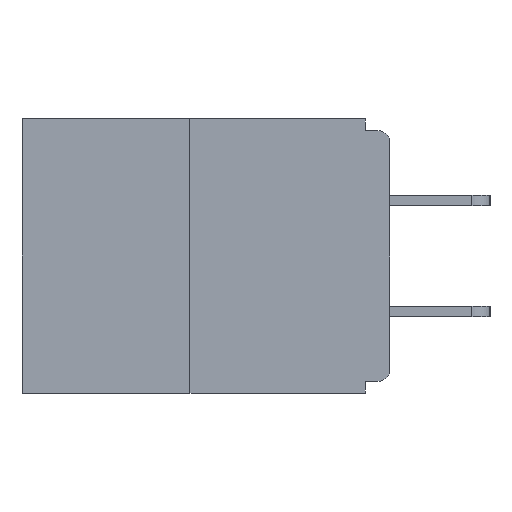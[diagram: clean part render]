
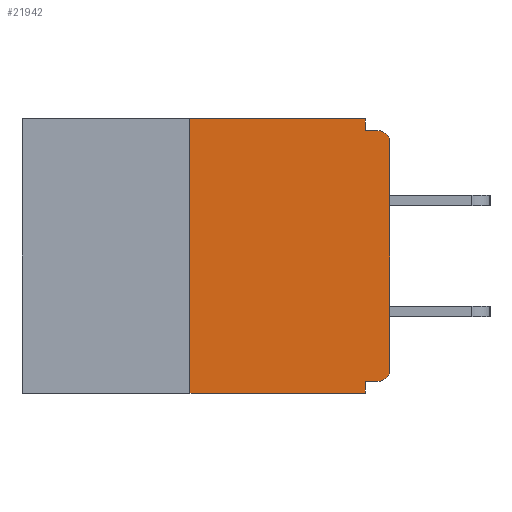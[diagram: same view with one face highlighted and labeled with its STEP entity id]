
A CAD part, left-side view. The second image highlights one B-rep face of the part: STEP entity #21942.
In plain terms, the highlighted planar face has unit normal (-1, 0, 0).
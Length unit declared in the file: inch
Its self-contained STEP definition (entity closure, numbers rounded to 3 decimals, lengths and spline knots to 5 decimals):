
#361 = VERTEX_POINT ( 'NONE', #21923 ) ;
#434 = VERTEX_POINT ( 'NONE', #30134 ) ;
#454 = ORIENTED_EDGE ( 'NONE', *, *, #24535, .T. ) ;
#1662 = ORIENTED_EDGE ( 'NONE', *, *, #8496, .T. ) ;
#2709 = EDGE_CURVE ( 'NONE', #361, #27647, #26786, .T. ) ;
#2742 = DIRECTION ( 'NONE',  ( 0., -1., 0. ) ) ;
#3403 = CARTESIAN_POINT ( 'NONE',  ( 0., 0.25, 0. ) ) ;
#4542 = VECTOR ( 'NONE', #15902, 39.37008 ) ;
#4855 = DIRECTION ( 'NONE',  ( 0., -1., 0. ) ) ;
#4894 = EDGE_CURVE ( 'NONE', #434, #29636, #6493, .T. ) ;
#4909 = DIRECTION ( 'NONE',  ( 0., 0., 1. ) ) ;
#4997 = VECTOR ( 'NONE', #4909, 39.37008 ) ;
#5574 = DIRECTION ( 'NONE',  ( 0., 0., -1. ) ) ;
#5601 = AXIS2_PLACEMENT_3D ( 'NONE', #25874, #28331, #13828 ) ;
#5640 = LINE ( 'NONE', #29507, #22577 ) ;
#5735 = ORIENTED_EDGE ( 'NONE', *, *, #2709, .F. ) ;
#6018 = VERTEX_POINT ( 'NONE', #18934 ) ;
#6100 = CARTESIAN_POINT ( 'NONE',  ( 0., 0.031, -0.343 ) ) ;
#6493 = LINE ( 'NONE', #15748, #4542 ) ;
#6708 = VECTOR ( 'NONE', #10724, 39.37008 ) ;
#7488 = VECTOR ( 'NONE', #20010, 39.37008 ) ;
#7684 = CARTESIAN_POINT ( 'NONE',  ( 0., 0.25, 0. ) ) ;
#8496 = EDGE_CURVE ( 'NONE', #24324, #27647, #19234, .T. ) ;
#10557 = EDGE_CURVE ( 'NONE', #6018, #22623, #15461, .T. ) ;
#10595 = CARTESIAN_POINT ( 'NONE',  ( 0., 0., 0. ) ) ;
#10724 = DIRECTION ( 'NONE',  ( 0., 0., -1. ) ) ;
#10898 = ORIENTED_EDGE ( 'NONE', *, *, #10557, .T. ) ;
#11642 = FACE_OUTER_BOUND ( 'NONE', #13571, .T. ) ;
#12263 = DIRECTION ( 'NONE',  ( 1., 0., 0. ) ) ;
#12884 = DIRECTION ( 'NONE',  ( 0., -1., 0. ) ) ;
#13135 = CARTESIAN_POINT ( 'NONE',  ( 0., 0.031, -0.015 ) ) ;
#13571 = EDGE_LOOP ( 'NONE', ( #16494, #15520, #1662, #5735, #25072, #22293, #454, #10898, #22321, #21813 ) ) ;
#13828 = DIRECTION ( 'NONE',  ( 0., 0., -1. ) ) ;
#13942 = CARTESIAN_POINT ( 'NONE',  ( 0., 0.46, 0. ) ) ;
#14294 = CARTESIAN_POINT ( 'NONE',  ( 0., 0.25, -0.343 ) ) ;
#14416 = PLANE ( 'NONE',  #18650 ) ;
#15041 = DIRECTION ( 'NONE',  ( 0., 1., 0. ) ) ;
#15461 = CIRCLE ( 'NONE', #5601, 0.015 ) ;
#15520 = ORIENTED_EDGE ( 'NONE', *, *, #24374, .F. ) ;
#15748 = CARTESIAN_POINT ( 'NONE',  ( 0., 0.031, 0. ) ) ;
#15755 = EDGE_CURVE ( 'NONE', #24033, #434, #21668, .T. ) ;
#15902 = DIRECTION ( 'NONE',  ( 0., 0., -1. ) ) ;
#16403 = EDGE_CURVE ( 'NONE', #29307, #30329, #26588, .T. ) ;
#16494 = ORIENTED_EDGE ( 'NONE', *, *, #15755, .F. ) ;
#16725 = DIRECTION ( 'NONE',  ( 0., 0., -1. ) ) ;
#17260 = VECTOR ( 'NONE', #4855, 39.37008 ) ;
#17502 = CARTESIAN_POINT ( 'NONE',  ( 0., 0.46, -0.343 ) ) ;
#17747 = CARTESIAN_POINT ( 'NONE',  ( 0., 0.015, -0.015 ) ) ;
#18650 = AXIS2_PLACEMENT_3D ( 'NONE', #13942, #12263, #16725 ) ;
#18934 = CARTESIAN_POINT ( 'NONE',  ( 0., 0., -0.03 ) ) ;
#19234 = LINE ( 'NONE', #17502, #23382 ) ;
#19475 = CARTESIAN_POINT ( 'NONE',  ( 0., 0.015, -0.313 ) ) ;
#19859 = LINE ( 'NONE', #10595, #7488 ) ;
#20010 = DIRECTION ( 'NONE',  ( 0., 0., 1. ) ) ;
#20741 = AXIS2_PLACEMENT_3D ( 'NONE', #19475, #28706, #5574 ) ;
#21358 = CARTESIAN_POINT ( 'NONE',  ( 0., 0.46, 0. ) ) ;
#21388 = CARTESIAN_POINT ( 'NONE',  ( 0., 0., -0.313 ) ) ;
#21668 = LINE ( 'NONE', #21358, #17260 ) ;
#21813 = ORIENTED_EDGE ( 'NONE', *, *, #4894, .F. ) ;
#21923 = CARTESIAN_POINT ( 'NONE',  ( 0., 0.031, -0.328 ) ) ;
#21942 = ADVANCED_FACE ( 'NONE', ( #11642 ), #14416, .F. ) ;
#21976 = CARTESIAN_POINT ( 'NONE',  ( 0., 0.031, -0.343 ) ) ;
#22051 = EDGE_CURVE ( 'NONE', #29307, #361, #24007, .T. ) ;
#22293 = ORIENTED_EDGE ( 'NONE', *, *, #16403, .T. ) ;
#22321 = ORIENTED_EDGE ( 'NONE', *, *, #27214, .F. ) ;
#22577 = VECTOR ( 'NONE', #12884, 39.37008 ) ;
#22623 = VERTEX_POINT ( 'NONE', #17747 ) ;
#23382 = VECTOR ( 'NONE', #2742, 39.37008 ) ;
#24007 = LINE ( 'NONE', #24462, #25070 ) ;
#24033 = VERTEX_POINT ( 'NONE', #3403 ) ;
#24324 = VERTEX_POINT ( 'NONE', #14294 ) ;
#24374 = EDGE_CURVE ( 'NONE', #24324, #24033, #28797, .T. ) ;
#24462 = CARTESIAN_POINT ( 'NONE',  ( 0., 0., -0.328 ) ) ;
#24535 = EDGE_CURVE ( 'NONE', #30329, #6018, #19859, .T. ) ;
#25070 = VECTOR ( 'NONE', #15041, 39.37008 ) ;
#25072 = ORIENTED_EDGE ( 'NONE', *, *, #22051, .F. ) ;
#25196 = CARTESIAN_POINT ( 'NONE',  ( 0., 0.015, -0.328 ) ) ;
#25874 = CARTESIAN_POINT ( 'NONE',  ( 0., 0.015, -0.03 ) ) ;
#26588 = CIRCLE ( 'NONE', #20741, 0.015 ) ;
#26786 = LINE ( 'NONE', #6100, #6708 ) ;
#27214 = EDGE_CURVE ( 'NONE', #29636, #22623, #5640, .T. ) ;
#27647 = VERTEX_POINT ( 'NONE', #21976 ) ;
#28331 = DIRECTION ( 'NONE',  ( -1., 0., 0. ) ) ;
#28706 = DIRECTION ( 'NONE',  ( -1., 0., 0. ) ) ;
#28797 = LINE ( 'NONE', #7684, #4997 ) ;
#29307 = VERTEX_POINT ( 'NONE', #25196 ) ;
#29507 = CARTESIAN_POINT ( 'NONE',  ( 0., 0., -0.015 ) ) ;
#29636 = VERTEX_POINT ( 'NONE', #13135 ) ;
#30134 = CARTESIAN_POINT ( 'NONE',  ( 0., 0.031, 0. ) ) ;
#30329 = VERTEX_POINT ( 'NONE', #21388 ) ;
